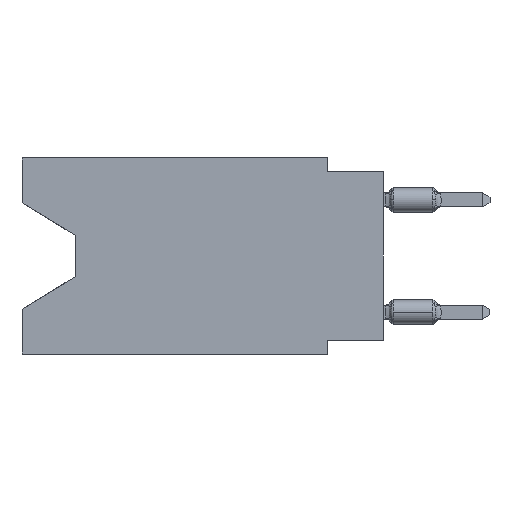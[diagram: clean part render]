
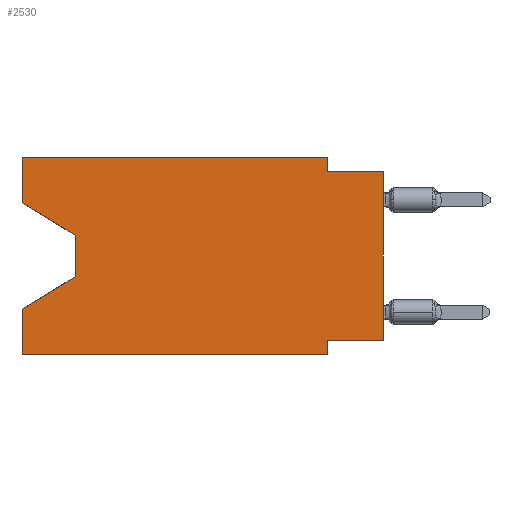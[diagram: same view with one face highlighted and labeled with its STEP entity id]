
A CAD part, left-side view. The second image highlights one B-rep face of the part: STEP entity #2530.
In plain terms, the highlighted planar face has unit normal (-1, 0, 0).
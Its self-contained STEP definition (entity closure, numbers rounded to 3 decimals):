
#164 = LINE ( 'NONE', #3292, #8219 ) ;
#170 = ORIENTED_EDGE ( 'NONE', *, *, #11598, .F. ) ;
#441 = VERTEX_POINT ( 'NONE', #9565 ) ;
#504 = DIRECTION ( 'NONE',  ( 0., 0., -1. ) ) ;
#531 = CARTESIAN_POINT ( 'NONE',  ( 0., 2.54, 0. ) ) ;
#683 = LINE ( 'NONE', #12005, #9738 ) ;
#804 = CARTESIAN_POINT ( 'NONE',  ( 0., 16.383, -8.89 ) ) ;
#817 = DIRECTION ( 'NONE',  ( 0., 0., 1. ) ) ;
#823 = AXIS2_PLACEMENT_3D ( 'NONE', #5767, #9971, #504 ) ;
#940 = CARTESIAN_POINT ( 'NONE',  ( 0., 16.383, 0. ) ) ;
#1114 = CARTESIAN_POINT ( 'NONE',  ( 0., 16.383, -8.89 ) ) ;
#1166 = CARTESIAN_POINT ( 'NONE',  ( 0., 2.54, -8.255 ) ) ;
#1956 = VERTEX_POINT ( 'NONE', #6823 ) ;
#2026 = ORIENTED_EDGE ( 'NONE', *, *, #9941, .F. ) ;
#2152 = LINE ( 'NONE', #5401, #10249 ) ;
#2530 = ADVANCED_FACE ( 'NONE', ( #3768 ), #7965, .F. ) ;
#2576 = LINE ( 'NONE', #11946, #12458 ) ;
#2824 = CARTESIAN_POINT ( 'NONE',  ( 0., 13.97, -3.505 ) ) ;
#3103 = LINE ( 'NONE', #804, #9837 ) ;
#3154 = CARTESIAN_POINT ( 'NONE',  ( 0., 0., -0.635 ) ) ;
#3201 = VECTOR ( 'NONE', #817, 1000. ) ;
#3292 = CARTESIAN_POINT ( 'NONE',  ( 0., 13.97, -5.385 ) ) ;
#3353 = EDGE_CURVE ( 'NONE', #12451, #6106, #12333, .T. ) ;
#3447 = LINE ( 'NONE', #8898, #9742 ) ;
#3768 = FACE_OUTER_BOUND ( 'NONE', #11489, .T. ) ;
#4069 = LINE ( 'NONE', #940, #7632 ) ;
#4213 = DIRECTION ( 'NONE',  ( 0., -1., 0. ) ) ;
#4763 = DIRECTION ( 'NONE',  ( 0., 0., -1. ) ) ;
#4967 = DIRECTION ( 'NONE',  ( 0., -1., 0. ) ) ;
#5136 = CARTESIAN_POINT ( 'NONE',  ( 0., 2.54, -0.635 ) ) ;
#5164 = DIRECTION ( 'NONE',  ( 0., 0.855, -0.519 ) ) ;
#5348 = EDGE_CURVE ( 'NONE', #6106, #10721, #164, .T. ) ;
#5401 = CARTESIAN_POINT ( 'NONE',  ( 0., 16.383, -2.038 ) ) ;
#5620 = VERTEX_POINT ( 'NONE', #5136 ) ;
#5767 = CARTESIAN_POINT ( 'NONE',  ( 0., 16.383, 0. ) ) ;
#5952 = LINE ( 'NONE', #11453, #3201 ) ;
#6106 = VERTEX_POINT ( 'NONE', #13648 ) ;
#6120 = VECTOR ( 'NONE', #6609, 1000. ) ;
#6195 = EDGE_CURVE ( 'NONE', #8379, #11063, #3447, .T. ) ;
#6385 = ORIENTED_EDGE ( 'NONE', *, *, #3353, .T. ) ;
#6596 = CARTESIAN_POINT ( 'NONE',  ( 0., 13.97, -3.505 ) ) ;
#6609 = DIRECTION ( 'NONE',  ( 0., 0., 1. ) ) ;
#6786 = CARTESIAN_POINT ( 'NONE',  ( 0., 16.383, -6.852 ) ) ;
#6823 = CARTESIAN_POINT ( 'NONE',  ( 0., 0., -8.255 ) ) ;
#6860 = VERTEX_POINT ( 'NONE', #1114 ) ;
#7027 = LINE ( 'NONE', #11221, #11979 ) ;
#7424 = ORIENTED_EDGE ( 'NONE', *, *, #8052, .F. ) ;
#7526 = ORIENTED_EDGE ( 'NONE', *, *, #9579, .T. ) ;
#7632 = VECTOR ( 'NONE', #4213, 1000. ) ;
#7661 = VERTEX_POINT ( 'NONE', #3154 ) ;
#7730 = DIRECTION ( 'NONE',  ( 0., 0., -1. ) ) ;
#7769 = EDGE_CURVE ( 'NONE', #9086, #441, #10941, .T. ) ;
#7778 = CARTESIAN_POINT ( 'NONE',  ( 0., 16.383, 0. ) ) ;
#7822 = ORIENTED_EDGE ( 'NONE', *, *, #11148, .F. ) ;
#7965 = PLANE ( 'NONE',  #823 ) ;
#7996 = LINE ( 'NONE', #531, #13253 ) ;
#8052 = EDGE_CURVE ( 'NONE', #5620, #7661, #2576, .T. ) ;
#8219 = VECTOR ( 'NONE', #5164, 1000. ) ;
#8379 = VERTEX_POINT ( 'NONE', #1166 ) ;
#8660 = ORIENTED_EDGE ( 'NONE', *, *, #5348, .T. ) ;
#8898 = CARTESIAN_POINT ( 'NONE',  ( 0., 2.54, -8.89 ) ) ;
#9059 = DIRECTION ( 'NONE',  ( 0., 0., 1. ) ) ;
#9086 = VERTEX_POINT ( 'NONE', #13323 ) ;
#9313 = DIRECTION ( 'NONE',  ( 0., 0., -1. ) ) ;
#9565 = CARTESIAN_POINT ( 'NONE',  ( 0., 16.383, 0. ) ) ;
#9579 = EDGE_CURVE ( 'NONE', #1956, #7661, #683, .T. ) ;
#9602 = DIRECTION ( 'NONE',  ( 0., -0.855, -0.519 ) ) ;
#9738 = VECTOR ( 'NONE', #9059, 1000. ) ;
#9742 = VECTOR ( 'NONE', #7730, 1000. ) ;
#9837 = VECTOR ( 'NONE', #4967, 1000. ) ;
#9941 = EDGE_CURVE ( 'NONE', #10723, #5620, #7996, .T. ) ;
#9971 = DIRECTION ( 'NONE',  ( 1., 0., 0. ) ) ;
#10249 = VECTOR ( 'NONE', #9602, 1000. ) ;
#10545 = ORIENTED_EDGE ( 'NONE', *, *, #11116, .T. ) ;
#10721 = VERTEX_POINT ( 'NONE', #6786 ) ;
#10723 = VERTEX_POINT ( 'NONE', #13185 ) ;
#10941 = LINE ( 'NONE', #7778, #6120 ) ;
#10971 = CARTESIAN_POINT ( 'NONE',  ( 0., 2.54, -8.89 ) ) ;
#11063 = VERTEX_POINT ( 'NONE', #10971 ) ;
#11116 = EDGE_CURVE ( 'NONE', #6860, #11063, #3103, .T. ) ;
#11148 = EDGE_CURVE ( 'NONE', #441, #10723, #4069, .T. ) ;
#11221 = CARTESIAN_POINT ( 'NONE',  ( 0., 0., -8.255 ) ) ;
#11285 = DIRECTION ( 'NONE',  ( 0., 1., 0. ) ) ;
#11453 = CARTESIAN_POINT ( 'NONE',  ( 0., 16.383, 0. ) ) ;
#11489 = EDGE_LOOP ( 'NONE', ( #12290, #6385, #8660, #11845, #10545, #13466, #170, #7526, #7424, #2026, #7822, #12988 ) ) ;
#11598 = EDGE_CURVE ( 'NONE', #1956, #8379, #7027, .T. ) ;
#11845 = ORIENTED_EDGE ( 'NONE', *, *, #12524, .F. ) ;
#11946 = CARTESIAN_POINT ( 'NONE',  ( 0., 0., -0.635 ) ) ;
#11979 = VECTOR ( 'NONE', #11285, 1000. ) ;
#12000 = EDGE_CURVE ( 'NONE', #9086, #12451, #2152, .T. ) ;
#12005 = CARTESIAN_POINT ( 'NONE',  ( 0., 0., 0. ) ) ;
#12143 = DIRECTION ( 'NONE',  ( 0., -1., 0. ) ) ;
#12290 = ORIENTED_EDGE ( 'NONE', *, *, #12000, .T. ) ;
#12299 = VECTOR ( 'NONE', #9313, 1000. ) ;
#12333 = LINE ( 'NONE', #2824, #12299 ) ;
#12451 = VERTEX_POINT ( 'NONE', #6596 ) ;
#12458 = VECTOR ( 'NONE', #12143, 1000. ) ;
#12524 = EDGE_CURVE ( 'NONE', #6860, #10721, #5952, .T. ) ;
#12988 = ORIENTED_EDGE ( 'NONE', *, *, #7769, .F. ) ;
#13185 = CARTESIAN_POINT ( 'NONE',  ( 0., 2.54, 0. ) ) ;
#13253 = VECTOR ( 'NONE', #4763, 1000. ) ;
#13323 = CARTESIAN_POINT ( 'NONE',  ( 0., 16.383, -2.038 ) ) ;
#13466 = ORIENTED_EDGE ( 'NONE', *, *, #6195, .F. ) ;
#13648 = CARTESIAN_POINT ( 'NONE',  ( 0., 13.97, -5.385 ) ) ;
